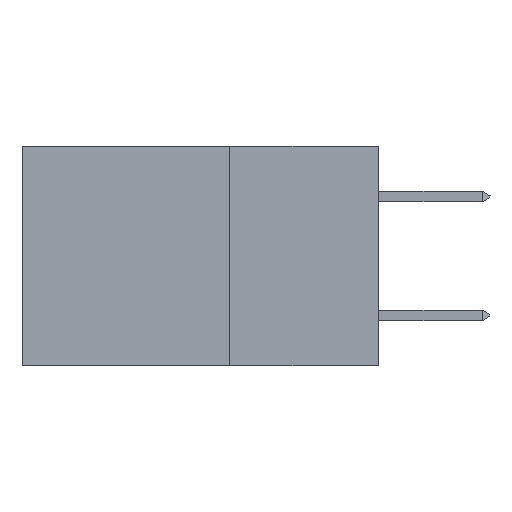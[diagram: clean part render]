
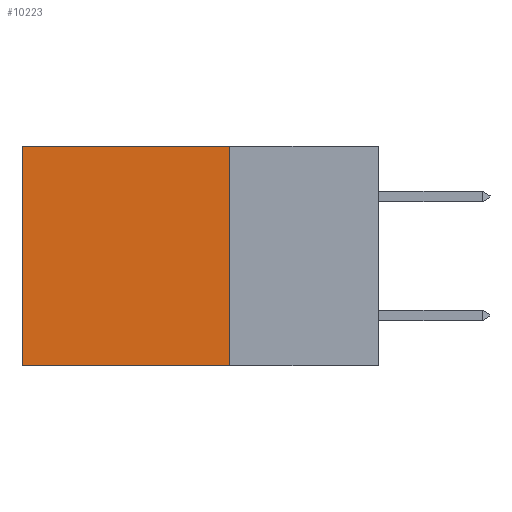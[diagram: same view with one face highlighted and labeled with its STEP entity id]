
A CAD part, left-side view. The second image highlights one B-rep face of the part: STEP entity #10223.
In plain terms, the highlighted planar face has unit normal (-1, 0, 0).
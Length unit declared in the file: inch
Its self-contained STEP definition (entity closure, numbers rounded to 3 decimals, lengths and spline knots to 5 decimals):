
#716 = CARTESIAN_POINT ( 'NONE',  ( 0.2615, 0.25, -0.37 ) ) ;
#807 = CARTESIAN_POINT ( 'NONE',  ( 0.2615, 0.25, 0. ) ) ;
#2277 = VECTOR ( 'NONE', #9791, 39.37008 ) ;
#2368 = VERTEX_POINT ( 'NONE', #807 ) ;
#2611 = DIRECTION ( 'NONE',  ( 0., 0., -1. ) ) ;
#2796 = DIRECTION ( 'NONE',  ( 0., 0., -1. ) ) ;
#3713 = VERTEX_POINT ( 'NONE', #13461 ) ;
#4316 = VECTOR ( 'NONE', #9851, 39.37008 ) ;
#4756 = CARTESIAN_POINT ( 'NONE',  ( 0.2615, 0.25, 0. ) ) ;
#5069 = DIRECTION ( 'NONE',  ( 1., 0., 0. ) ) ;
#5130 = CARTESIAN_POINT ( 'NONE',  ( 0.2615, 0.6, -0.37 ) ) ;
#5406 = VERTEX_POINT ( 'NONE', #716 ) ;
#6312 = CARTESIAN_POINT ( 'NONE',  ( 0.2615, 0.6, 0. ) ) ;
#6795 = EDGE_LOOP ( 'NONE', ( #10023, #8011, #13332, #8332 ) ) ;
#7112 = EDGE_CURVE ( 'NONE', #2368, #14407, #12263, .T. ) ;
#7637 = LINE ( 'NONE', #5130, #12448 ) ;
#8011 = ORIENTED_EDGE ( 'NONE', *, *, #15746, .F. ) ;
#8332 = ORIENTED_EDGE ( 'NONE', *, *, #7112, .T. ) ;
#8468 = CARTESIAN_POINT ( 'NONE',  ( 0.2615, 0.25, -0.37 ) ) ;
#8551 = LINE ( 'NONE', #8468, #8704 ) ;
#8704 = VECTOR ( 'NONE', #15015, 39.37008 ) ;
#9791 = DIRECTION ( 'NONE',  ( 0., 0., -1. ) ) ;
#9851 = DIRECTION ( 'NONE',  ( 0., 1., 0. ) ) ;
#10023 = ORIENTED_EDGE ( 'NONE', *, *, #15853, .T. ) ;
#10223 = ADVANCED_FACE ( 'NONE', ( #15453 ), #15523, .F. ) ;
#11546 = AXIS2_PLACEMENT_3D ( 'NONE', #14278, #5069, #2796 ) ;
#12263 = LINE ( 'NONE', #4756, #4316 ) ;
#12448 = VECTOR ( 'NONE', #2611, 39.37008 ) ;
#13332 = ORIENTED_EDGE ( 'NONE', *, *, #16248, .F. ) ;
#13461 = CARTESIAN_POINT ( 'NONE',  ( 0.2615, 0.6, -0.37 ) ) ;
#13735 = CARTESIAN_POINT ( 'NONE',  ( 0.2615, 0.25, -0.37 ) ) ;
#14278 = CARTESIAN_POINT ( 'NONE',  ( 0.2615, 0.25, -0.37 ) ) ;
#14407 = VERTEX_POINT ( 'NONE', #6312 ) ;
#15015 = DIRECTION ( 'NONE',  ( 0., 1., 0. ) ) ;
#15453 = FACE_OUTER_BOUND ( 'NONE', #6795, .T. ) ;
#15523 = PLANE ( 'NONE',  #11546 ) ;
#15746 = EDGE_CURVE ( 'NONE', #5406, #3713, #8551, .T. ) ;
#15853 = EDGE_CURVE ( 'NONE', #14407, #3713, #7637, .T. ) ;
#16072 = LINE ( 'NONE', #13735, #2277 ) ;
#16248 = EDGE_CURVE ( 'NONE', #2368, #5406, #16072, .T. ) ;
